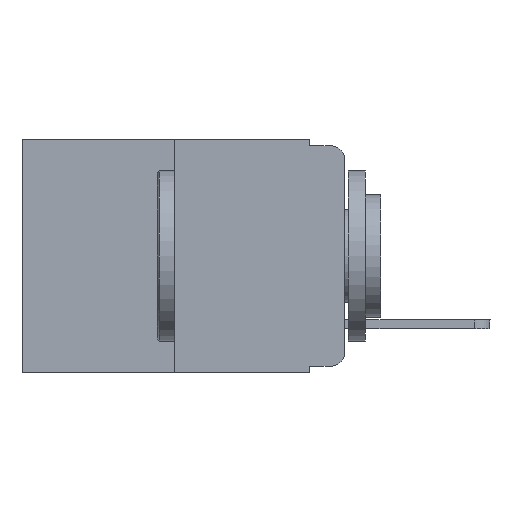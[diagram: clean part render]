
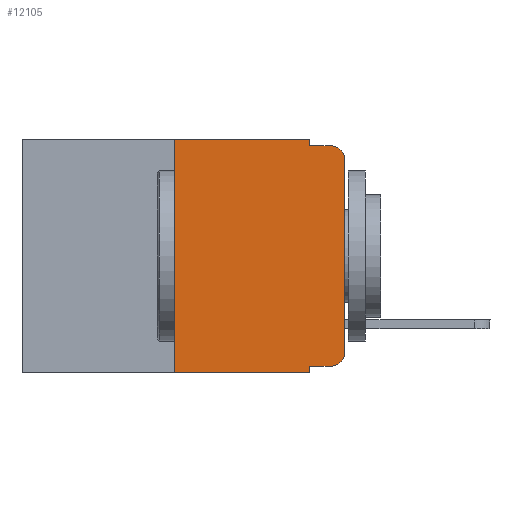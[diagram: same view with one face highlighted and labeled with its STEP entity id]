
A CAD part, left-side view. The second image highlights one B-rep face of the part: STEP entity #12105.
In plain terms, the highlighted planar face has unit normal (-1, 0, 0).
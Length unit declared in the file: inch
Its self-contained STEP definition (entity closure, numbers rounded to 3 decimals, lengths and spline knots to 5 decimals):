
#143 = CARTESIAN_POINT ( 'NONE',  ( 0., 0.473, 0. ) ) ;
#175 = DIRECTION ( 'NONE',  ( -1., 0., 0. ) ) ;
#301 = DIRECTION ( 'NONE',  ( 0., 0., 1. ) ) ;
#442 = VECTOR ( 'NONE', #14312, 39.37008 ) ;
#694 = LINE ( 'NONE', #15799, #15675 ) ;
#900 = DIRECTION ( 'NONE',  ( 1., 0., 0. ) ) ;
#965 = EDGE_CURVE ( 'NONE', #14627, #4883, #5344, .T. ) ;
#1108 = VECTOR ( 'NONE', #14523, 39.37008 ) ;
#1342 = ORIENTED_EDGE ( 'NONE', *, *, #15129, .T. ) ;
#1562 = LINE ( 'NONE', #143, #11333 ) ;
#1900 = CARTESIAN_POINT ( 'NONE',  ( 0., 0.051, 0. ) ) ;
#2391 = CARTESIAN_POINT ( 'NONE',  ( 0., 0.25, 0. ) ) ;
#2797 = EDGE_CURVE ( 'NONE', #5090, #2985, #15901, .T. ) ;
#2951 = AXIS2_PLACEMENT_3D ( 'NONE', #8142, #175, #13274 ) ;
#2985 = VERTEX_POINT ( 'NONE', #4363 ) ;
#3009 = EDGE_LOOP ( 'NONE', ( #8669, #9211, #6628, #8779, #3358, #13818, #15328, #15940, #1342, #14768 ) ) ;
#3028 = CIRCLE ( 'NONE', #2951, 0.02 ) ;
#3137 = EDGE_CURVE ( 'NONE', #8709, #2985, #694, .T. ) ;
#3224 = LINE ( 'NONE', #4687, #9449 ) ;
#3358 = ORIENTED_EDGE ( 'NONE', *, *, #10330, .F. ) ;
#3553 = CARTESIAN_POINT ( 'NONE',  ( 0., 0.051, -0.343 ) ) ;
#3656 = CARTESIAN_POINT ( 'NONE',  ( 0., 0.473, -0.343 ) ) ;
#4363 = CARTESIAN_POINT ( 'NONE',  ( 0., 0.02, -0.01 ) ) ;
#4492 = AXIS2_PLACEMENT_3D ( 'NONE', #9974, #900, #14168 ) ;
#4687 = CARTESIAN_POINT ( 'NONE',  ( 0., 0.051, 0. ) ) ;
#4715 = AXIS2_PLACEMENT_3D ( 'NONE', #6752, #16036, #17088 ) ;
#4883 = VERTEX_POINT ( 'NONE', #15590 ) ;
#5057 = CARTESIAN_POINT ( 'NONE',  ( 0., 0.02, -0.333 ) ) ;
#5063 = CARTESIAN_POINT ( 'NONE',  ( 0., 0.051, -0.01 ) ) ;
#5090 = VERTEX_POINT ( 'NONE', #7576 ) ;
#5344 = LINE ( 'NONE', #2391, #16782 ) ;
#5477 = DIRECTION ( 'NONE',  ( 0., -1., 0. ) ) ;
#6628 = ORIENTED_EDGE ( 'NONE', *, *, #3137, .F. ) ;
#6752 = CARTESIAN_POINT ( 'NONE',  ( 0., 0.02, -0.03 ) ) ;
#6816 = CARTESIAN_POINT ( 'NONE',  ( 0., 0., 0. ) ) ;
#6855 = EDGE_CURVE ( 'NONE', #15208, #5090, #8951, .T. ) ;
#6982 = DIRECTION ( 'NONE',  ( 0., -1., 0. ) ) ;
#7198 = DIRECTION ( 'NONE',  ( 0., 0., -1. ) ) ;
#7292 = PLANE ( 'NONE',  #4492 ) ;
#7308 = CARTESIAN_POINT ( 'NONE',  ( 0., 0., -0.313 ) ) ;
#7576 = CARTESIAN_POINT ( 'NONE',  ( 0., 0., -0.03 ) ) ;
#7753 = CARTESIAN_POINT ( 'NONE',  ( 0., 0.051, -0.333 ) ) ;
#7757 = LINE ( 'NONE', #11216, #1108 ) ;
#8142 = CARTESIAN_POINT ( 'NONE',  ( 0., 0.02, -0.313 ) ) ;
#8669 = ORIENTED_EDGE ( 'NONE', *, *, #6855, .T. ) ;
#8709 = VERTEX_POINT ( 'NONE', #5063 ) ;
#8779 = ORIENTED_EDGE ( 'NONE', *, *, #13387, .F. ) ;
#8951 = LINE ( 'NONE', #6816, #15009 ) ;
#9211 = ORIENTED_EDGE ( 'NONE', *, *, #2797, .T. ) ;
#9449 = VECTOR ( 'NONE', #7198, 39.37008 ) ;
#9974 = CARTESIAN_POINT ( 'NONE',  ( 0., 0.473, 0. ) ) ;
#10330 = EDGE_CURVE ( 'NONE', #4883, #15870, #1562, .T. ) ;
#10808 = VERTEX_POINT ( 'NONE', #7753 ) ;
#11216 = CARTESIAN_POINT ( 'NONE',  ( 0., 0.051, 0. ) ) ;
#11333 = VECTOR ( 'NONE', #5477, 39.37008 ) ;
#11685 = DIRECTION ( 'NONE',  ( 0., 0., 1. ) ) ;
#12096 = DIRECTION ( 'NONE',  ( 0., -1., 0. ) ) ;
#12105 = ADVANCED_FACE ( 'NONE', ( #12743 ), #7292, .F. ) ;
#12328 = LINE ( 'NONE', #14959, #16875 ) ;
#12743 = FACE_OUTER_BOUND ( 'NONE', #3009, .T. ) ;
#12870 = VERTEX_POINT ( 'NONE', #3553 ) ;
#13120 = EDGE_CURVE ( 'NONE', #16765, #15208, #3028, .T. ) ;
#13160 = LINE ( 'NONE', #3656, #442 ) ;
#13274 = DIRECTION ( 'NONE',  ( 0., 0., -1. ) ) ;
#13387 = EDGE_CURVE ( 'NONE', #15870, #8709, #3224, .T. ) ;
#13818 = ORIENTED_EDGE ( 'NONE', *, *, #965, .F. ) ;
#14168 = DIRECTION ( 'NONE',  ( 0., 0., -1. ) ) ;
#14312 = DIRECTION ( 'NONE',  ( 0., -1., 0. ) ) ;
#14523 = DIRECTION ( 'NONE',  ( 0., 0., -1. ) ) ;
#14627 = VERTEX_POINT ( 'NONE', #16503 ) ;
#14768 = ORIENTED_EDGE ( 'NONE', *, *, #13120, .T. ) ;
#14829 = EDGE_CURVE ( 'NONE', #10808, #12870, #7757, .T. ) ;
#14959 = CARTESIAN_POINT ( 'NONE',  ( 0., 0.051, -0.333 ) ) ;
#15009 = VECTOR ( 'NONE', #301, 39.37008 ) ;
#15129 = EDGE_CURVE ( 'NONE', #10808, #16765, #12328, .T. ) ;
#15208 = VERTEX_POINT ( 'NONE', #7308 ) ;
#15328 = ORIENTED_EDGE ( 'NONE', *, *, #15372, .T. ) ;
#15372 = EDGE_CURVE ( 'NONE', #14627, #12870, #13160, .T. ) ;
#15590 = CARTESIAN_POINT ( 'NONE',  ( 0., 0.25, 0. ) ) ;
#15675 = VECTOR ( 'NONE', #12096, 39.37008 ) ;
#15799 = CARTESIAN_POINT ( 'NONE',  ( 0., 0.051, -0.01 ) ) ;
#15870 = VERTEX_POINT ( 'NONE', #1900 ) ;
#15901 = CIRCLE ( 'NONE', #4715, 0.02 ) ;
#15940 = ORIENTED_EDGE ( 'NONE', *, *, #14829, .F. ) ;
#16036 = DIRECTION ( 'NONE',  ( -1., 0., 0. ) ) ;
#16503 = CARTESIAN_POINT ( 'NONE',  ( 0., 0.25, -0.343 ) ) ;
#16765 = VERTEX_POINT ( 'NONE', #5057 ) ;
#16782 = VECTOR ( 'NONE', #11685, 39.37008 ) ;
#16875 = VECTOR ( 'NONE', #6982, 39.37008 ) ;
#17088 = DIRECTION ( 'NONE',  ( 0., 0., -1. ) ) ;
